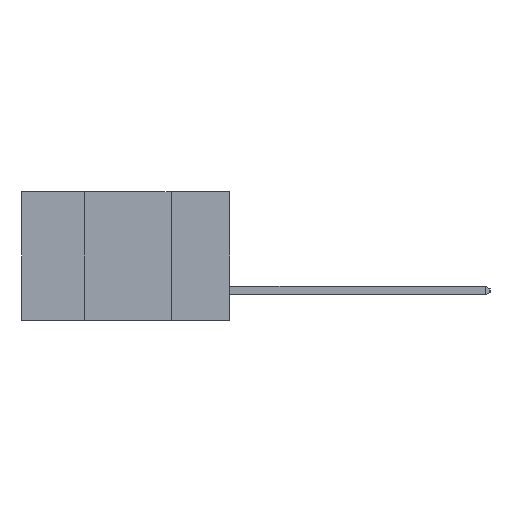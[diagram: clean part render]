
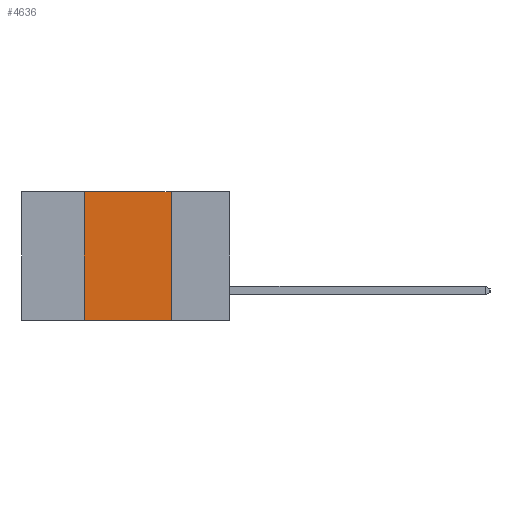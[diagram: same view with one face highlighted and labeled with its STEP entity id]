
A CAD part, left-side view. The second image highlights one B-rep face of the part: STEP entity #4636.
In plain terms, the highlighted planar face has unit normal (-1, 0, 0).
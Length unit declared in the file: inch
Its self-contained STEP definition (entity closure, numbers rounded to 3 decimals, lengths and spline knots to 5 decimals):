
#333 = FACE_OUTER_BOUND ( 'NONE', #3171, .T. ) ;
#443 = CARTESIAN_POINT ( 'NONE',  ( 0., 0.42, -0.37 ) ) ;
#624 = CARTESIAN_POINT ( 'NONE',  ( 0., 0.17, 0. ) ) ;
#877 = VERTEX_POINT ( 'NONE', #3325 ) ;
#1661 = VERTEX_POINT ( 'NONE', #3809 ) ;
#2120 = VERTEX_POINT ( 'NONE', #624 ) ;
#2602 = CARTESIAN_POINT ( 'NONE',  ( 0., 0.6, 0. ) ) ;
#2735 = DIRECTION ( 'NONE',  ( 0., 0., -1. ) ) ;
#2809 = VECTOR ( 'NONE', #3903, 39.37008 ) ;
#3171 = EDGE_LOOP ( 'NONE', ( #8908, #3545, #11963, #3887 ) ) ;
#3325 = CARTESIAN_POINT ( 'NONE',  ( 0., 0.17, -0.37 ) ) ;
#3364 = VECTOR ( 'NONE', #8750, 39.37008 ) ;
#3545 = ORIENTED_EDGE ( 'NONE', *, *, #6553, .F. ) ;
#3615 = VECTOR ( 'NONE', #2735, 39.37008 ) ;
#3809 = CARTESIAN_POINT ( 'NONE',  ( 0., 0.42, -0.37 ) ) ;
#3887 = ORIENTED_EDGE ( 'NONE', *, *, #5103, .T. ) ;
#3903 = DIRECTION ( 'NONE',  ( 0., 0., 1. ) ) ;
#4636 = ADVANCED_FACE ( 'NONE', ( #333 ), #9077, .F. ) ;
#4846 = DIRECTION ( 'NONE',  ( 1., 0., 0. ) ) ;
#4891 = CARTESIAN_POINT ( 'NONE',  ( 0., 0.6, 0. ) ) ;
#5103 = EDGE_CURVE ( 'NONE', #1661, #877, #11803, .T. ) ;
#5407 = LINE ( 'NONE', #443, #2809 ) ;
#5847 = EDGE_CURVE ( 'NONE', #1661, #6743, #5407, .T. ) ;
#6156 = LINE ( 'NONE', #12250, #3615 ) ;
#6553 = EDGE_CURVE ( 'NONE', #6743, #2120, #12210, .T. ) ;
#6686 = VECTOR ( 'NONE', #11163, 39.37008 ) ;
#6743 = VERTEX_POINT ( 'NONE', #9381 ) ;
#7259 = EDGE_CURVE ( 'NONE', #2120, #877, #6156, .T. ) ;
#8467 = AXIS2_PLACEMENT_3D ( 'NONE', #2602, #4846, #12179 ) ;
#8750 = DIRECTION ( 'NONE',  ( 0., -1., 0. ) ) ;
#8908 = ORIENTED_EDGE ( 'NONE', *, *, #7259, .F. ) ;
#9077 = PLANE ( 'NONE',  #8467 ) ;
#9381 = CARTESIAN_POINT ( 'NONE',  ( 0., 0.42, 0. ) ) ;
#11163 = DIRECTION ( 'NONE',  ( 0., -1., 0. ) ) ;
#11803 = LINE ( 'NONE', #13784, #3364 ) ;
#11963 = ORIENTED_EDGE ( 'NONE', *, *, #5847, .F. ) ;
#12179 = DIRECTION ( 'NONE',  ( 0., 0., -1. ) ) ;
#12210 = LINE ( 'NONE', #4891, #6686 ) ;
#12250 = CARTESIAN_POINT ( 'NONE',  ( 0., 0.17, -0.37 ) ) ;
#13784 = CARTESIAN_POINT ( 'NONE',  ( 0., 0.6, -0.37 ) ) ;
